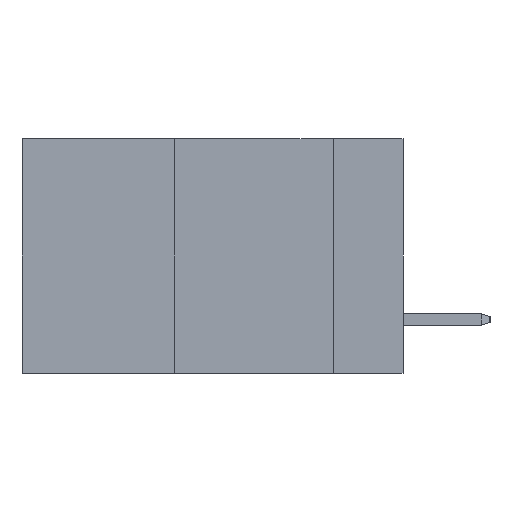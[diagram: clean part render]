
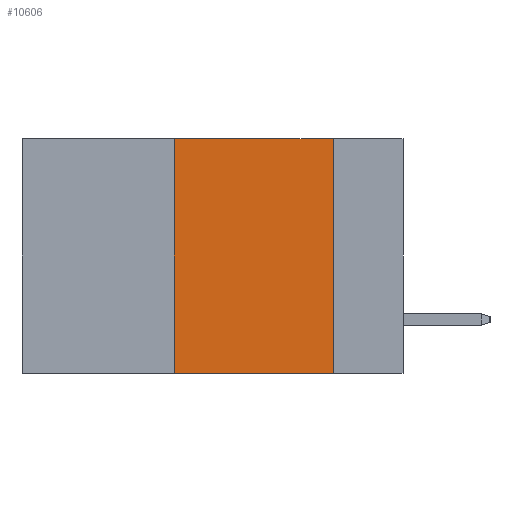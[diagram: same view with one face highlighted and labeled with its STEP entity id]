
A CAD part, left-side view. The second image highlights one B-rep face of the part: STEP entity #10606.
In plain terms, the highlighted planar face has unit normal (-1, 0, 0).
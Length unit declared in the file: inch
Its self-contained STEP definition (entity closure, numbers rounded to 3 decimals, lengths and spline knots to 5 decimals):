
#204 = VERTEX_POINT ( 'NONE', #754 ) ;
#754 = CARTESIAN_POINT ( 'NONE',  ( 0., 0.11, 0. ) ) ;
#1508 = CARTESIAN_POINT ( 'NONE',  ( 0., 0.36, -0.37 ) ) ;
#2092 = VECTOR ( 'NONE', #11393, 39.37008 ) ;
#2635 = VECTOR ( 'NONE', #19109, 39.37008 ) ;
#2667 = LINE ( 'NONE', #9031, #2092 ) ;
#2824 = DIRECTION ( 'NONE',  ( 0., 0., 1. ) ) ;
#3014 = CARTESIAN_POINT ( 'NONE',  ( 0., 0.11, -0.37 ) ) ;
#3254 = LINE ( 'NONE', #15965, #2635 ) ;
#3484 = PLANE ( 'NONE',  #18394 ) ;
#3811 = EDGE_CURVE ( 'NONE', #13840, #9907, #20358, .T. ) ;
#4721 = ORIENTED_EDGE ( 'NONE', *, *, #18351, .F. ) ;
#5148 = DIRECTION ( 'NONE',  ( 0., 0., -1. ) ) ;
#5714 = ORIENTED_EDGE ( 'NONE', *, *, #9245, .F. ) ;
#6714 = DIRECTION ( 'NONE',  ( 1., 0., 0. ) ) ;
#6887 = DIRECTION ( 'NONE',  ( 0., -1., 0. ) ) ;
#6988 = CARTESIAN_POINT ( 'NONE',  ( 0., 0.6, 0. ) ) ;
#9031 = CARTESIAN_POINT ( 'NONE',  ( 0., 0.6, -0.37 ) ) ;
#9245 = EDGE_CURVE ( 'NONE', #9907, #204, #13451, .T. ) ;
#9538 = VERTEX_POINT ( 'NONE', #3014 ) ;
#9804 = ORIENTED_EDGE ( 'NONE', *, *, #3811, .F. ) ;
#9843 = CARTESIAN_POINT ( 'NONE',  ( 0., 0.6, 0. ) ) ;
#9907 = VERTEX_POINT ( 'NONE', #11937 ) ;
#10606 = ADVANCED_FACE ( 'NONE', ( #17777 ), #3484, .F. ) ;
#11393 = DIRECTION ( 'NONE',  ( 0., -1., 0. ) ) ;
#11937 = CARTESIAN_POINT ( 'NONE',  ( 0., 0.36, 0. ) ) ;
#12666 = VECTOR ( 'NONE', #6887, 39.37008 ) ;
#13451 = LINE ( 'NONE', #6988, #12666 ) ;
#13629 = ORIENTED_EDGE ( 'NONE', *, *, #16373, .T. ) ;
#13840 = VERTEX_POINT ( 'NONE', #1508 ) ;
#15643 = VECTOR ( 'NONE', #2824, 39.37008 ) ;
#15748 = CARTESIAN_POINT ( 'NONE',  ( 0., 0.36, 0. ) ) ;
#15965 = CARTESIAN_POINT ( 'NONE',  ( 0., 0.11, 0. ) ) ;
#16373 = EDGE_CURVE ( 'NONE', #13840, #9538, #2667, .T. ) ;
#17777 = FACE_OUTER_BOUND ( 'NONE', #18131, .T. ) ;
#18131 = EDGE_LOOP ( 'NONE', ( #4721, #5714, #9804, #13629 ) ) ;
#18351 = EDGE_CURVE ( 'NONE', #204, #9538, #3254, .T. ) ;
#18394 = AXIS2_PLACEMENT_3D ( 'NONE', #9843, #6714, #5148 ) ;
#19109 = DIRECTION ( 'NONE',  ( 0., 0., -1. ) ) ;
#20358 = LINE ( 'NONE', #15748, #15643 ) ;
